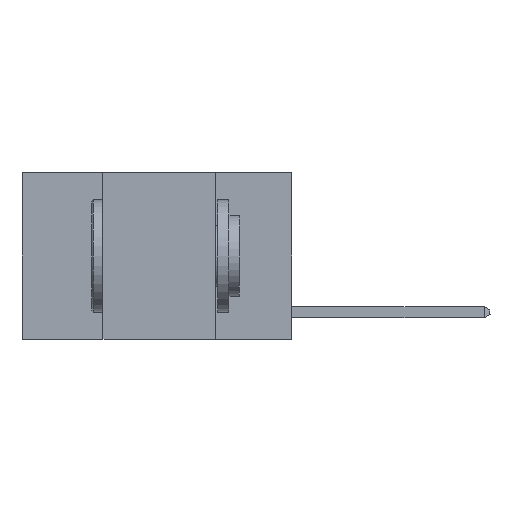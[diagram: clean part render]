
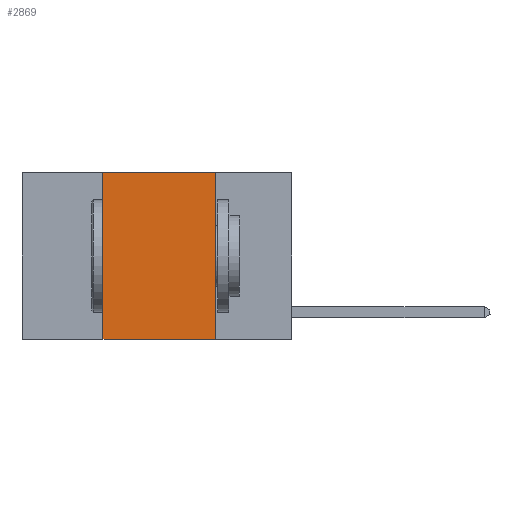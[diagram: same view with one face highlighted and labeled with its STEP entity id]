
A CAD part, left-side view. The second image highlights one B-rep face of the part: STEP entity #2869.
In plain terms, the highlighted planar face has unit normal (-1, 0, 0).
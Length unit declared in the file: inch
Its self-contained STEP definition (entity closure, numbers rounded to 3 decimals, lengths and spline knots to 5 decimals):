
#35 = EDGE_CURVE ( 'NONE', #6040, #4406, #1791, .T. ) ;
#134 = FACE_OUTER_BOUND ( 'NONE', #1674, .T. ) ;
#822 = CARTESIAN_POINT ( 'NONE',  ( 0., 0.17, 0. ) ) ;
#1002 = CARTESIAN_POINT ( 'NONE',  ( 0., 0.6, -0.37 ) ) ;
#1087 = ORIENTED_EDGE ( 'NONE', *, *, #35, .T. ) ;
#1135 = DIRECTION ( 'NONE',  ( 0., -1., 0. ) ) ;
#1217 = AXIS2_PLACEMENT_3D ( 'NONE', #2744, #8499, #7934 ) ;
#1223 = CARTESIAN_POINT ( 'NONE',  ( 0., 0.42, 0. ) ) ;
#1674 = EDGE_LOOP ( 'NONE', ( #6305, #2537, #4501, #1087 ) ) ;
#1791 = LINE ( 'NONE', #1002, #7435 ) ;
#1921 = DIRECTION ( 'NONE',  ( 0., 0., 1. ) ) ;
#2152 = VECTOR ( 'NONE', #1921, 39.37008 ) ;
#2215 = CARTESIAN_POINT ( 'NONE',  ( 0., 0.42, -0.37 ) ) ;
#2537 = ORIENTED_EDGE ( 'NONE', *, *, #2677, .F. ) ;
#2605 = CARTESIAN_POINT ( 'NONE',  ( 0., 0.6, 0. ) ) ;
#2677 = EDGE_CURVE ( 'NONE', #5305, #8583, #5716, .T. ) ;
#2744 = CARTESIAN_POINT ( 'NONE',  ( 0., 0.6, 0. ) ) ;
#2869 = ADVANCED_FACE ( 'NONE', ( #134 ), #5814, .F. ) ;
#2963 = DIRECTION ( 'NONE',  ( 0., 0., -1. ) ) ;
#3046 = VECTOR ( 'NONE', #2963, 39.37008 ) ;
#4406 = VERTEX_POINT ( 'NONE', #6905 ) ;
#4501 = ORIENTED_EDGE ( 'NONE', *, *, #8444, .F. ) ;
#4524 = DIRECTION ( 'NONE',  ( 0., -1., 0. ) ) ;
#5305 = VERTEX_POINT ( 'NONE', #5912 ) ;
#5716 = LINE ( 'NONE', #2605, #9202 ) ;
#5814 = PLANE ( 'NONE',  #1217 ) ;
#5912 = CARTESIAN_POINT ( 'NONE',  ( 0., 0.42, 0. ) ) ;
#6040 = VERTEX_POINT ( 'NONE', #2215 ) ;
#6305 = ORIENTED_EDGE ( 'NONE', *, *, #8745, .F. ) ;
#6905 = CARTESIAN_POINT ( 'NONE',  ( 0., 0.17, -0.37 ) ) ;
#7213 = CARTESIAN_POINT ( 'NONE',  ( 0., 0.17, 0. ) ) ;
#7435 = VECTOR ( 'NONE', #4524, 39.37008 ) ;
#7934 = DIRECTION ( 'NONE',  ( 0., 0., -1. ) ) ;
#8008 = LINE ( 'NONE', #1223, #2152 ) ;
#8444 = EDGE_CURVE ( 'NONE', #6040, #5305, #8008, .T. ) ;
#8499 = DIRECTION ( 'NONE',  ( 1., 0., 0. ) ) ;
#8583 = VERTEX_POINT ( 'NONE', #7213 ) ;
#8745 = EDGE_CURVE ( 'NONE', #8583, #4406, #9040, .T. ) ;
#9040 = LINE ( 'NONE', #822, #3046 ) ;
#9202 = VECTOR ( 'NONE', #1135, 39.37008 ) ;
